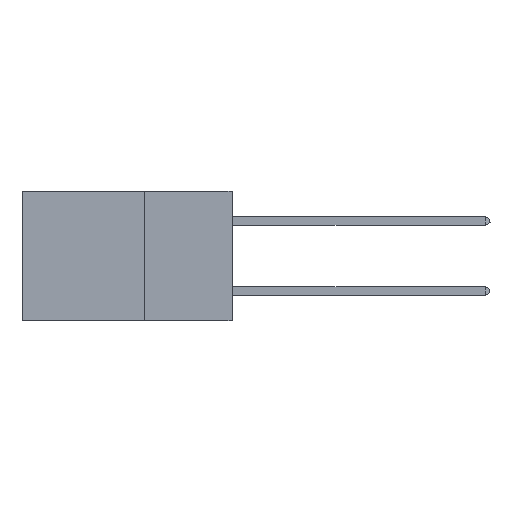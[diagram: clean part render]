
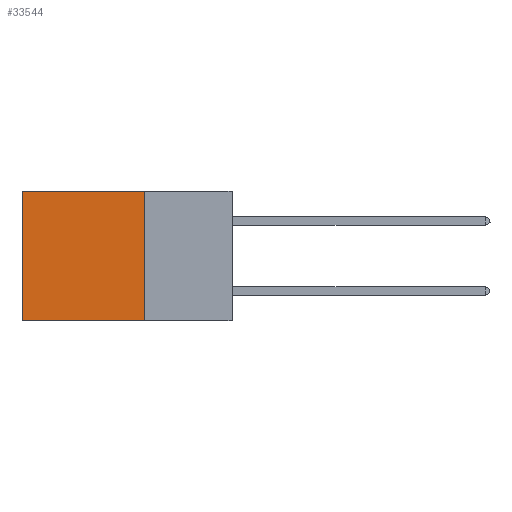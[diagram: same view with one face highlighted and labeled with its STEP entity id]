
A CAD part, left-side view. The second image highlights one B-rep face of the part: STEP entity #33544.
In plain terms, the highlighted planar face has unit normal (-1, 0, 0).
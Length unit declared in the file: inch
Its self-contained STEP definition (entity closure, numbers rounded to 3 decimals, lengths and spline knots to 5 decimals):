
#466 = CARTESIAN_POINT ( 'NONE',  ( 0.2875, 0.25, 0. ) ) ;
#1503 = DIRECTION ( 'NONE',  ( 1., 0., 0. ) ) ;
#2837 = EDGE_CURVE ( 'NONE', #16611, #35384, #21919, .T. ) ;
#2863 = LINE ( 'NONE', #15041, #17039 ) ;
#3520 = DIRECTION ( 'NONE',  ( 0., 1., 0. ) ) ;
#4257 = ORIENTED_EDGE ( 'NONE', *, *, #2837, .T. ) ;
#4682 = ORIENTED_EDGE ( 'NONE', *, *, #18660, .F. ) ;
#4981 = EDGE_CURVE ( 'NONE', #12244, #16611, #2863, .T. ) ;
#5864 = ORIENTED_EDGE ( 'NONE', *, *, #19652, .F. ) ;
#6273 = ORIENTED_EDGE ( 'NONE', *, *, #4981, .T. ) ;
#6308 = CARTESIAN_POINT ( 'NONE',  ( 0.2875, 0.6, 0. ) ) ;
#9098 = CARTESIAN_POINT ( 'NONE',  ( 0.2875, 0.25, -0.37 ) ) ;
#9104 = LINE ( 'NONE', #466, #19723 ) ;
#11812 = DIRECTION ( 'NONE',  ( 0., 0., -1. ) ) ;
#12109 = DIRECTION ( 'NONE',  ( 0., 0., -1. ) ) ;
#12244 = VERTEX_POINT ( 'NONE', #25998 ) ;
#13286 = FACE_OUTER_BOUND ( 'NONE', #30575, .T. ) ;
#14954 = VECTOR ( 'NONE', #18937, 39.37008 ) ;
#15041 = CARTESIAN_POINT ( 'NONE',  ( 0.2875, 0.25, 0. ) ) ;
#15716 = CARTESIAN_POINT ( 'NONE',  ( 0.2875, 0.6, 0. ) ) ;
#16611 = VERTEX_POINT ( 'NONE', #15716 ) ;
#17039 = VECTOR ( 'NONE', #3520, 39.37008 ) ;
#18660 = EDGE_CURVE ( 'NONE', #21128, #35384, #25127, .T. ) ;
#18937 = DIRECTION ( 'NONE',  ( 0., 1., 0. ) ) ;
#19652 = EDGE_CURVE ( 'NONE', #12244, #21128, #9104, .T. ) ;
#19723 = VECTOR ( 'NONE', #11812, 39.37008 ) ;
#21128 = VERTEX_POINT ( 'NONE', #31936 ) ;
#21287 = DIRECTION ( 'NONE',  ( 0., 0., -1. ) ) ;
#21919 = LINE ( 'NONE', #6308, #32929 ) ;
#23071 = AXIS2_PLACEMENT_3D ( 'NONE', #23766, #1503, #21287 ) ;
#23766 = CARTESIAN_POINT ( 'NONE',  ( 0.2875, 0.25, 0. ) ) ;
#25127 = LINE ( 'NONE', #9098, #14954 ) ;
#25998 = CARTESIAN_POINT ( 'NONE',  ( 0.2875, 0.25, 0. ) ) ;
#26594 = PLANE ( 'NONE',  #23071 ) ;
#29334 = CARTESIAN_POINT ( 'NONE',  ( 0.2875, 0.6, -0.37 ) ) ;
#30575 = EDGE_LOOP ( 'NONE', ( #4257, #4682, #5864, #6273 ) ) ;
#31936 = CARTESIAN_POINT ( 'NONE',  ( 0.2875, 0.25, -0.37 ) ) ;
#32929 = VECTOR ( 'NONE', #12109, 39.37008 ) ;
#33544 = ADVANCED_FACE ( 'NONE', ( #13286 ), #26594, .F. ) ;
#35384 = VERTEX_POINT ( 'NONE', #29334 ) ;
